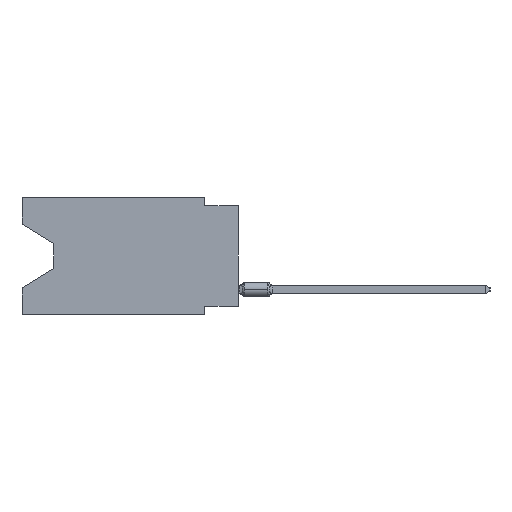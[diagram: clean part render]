
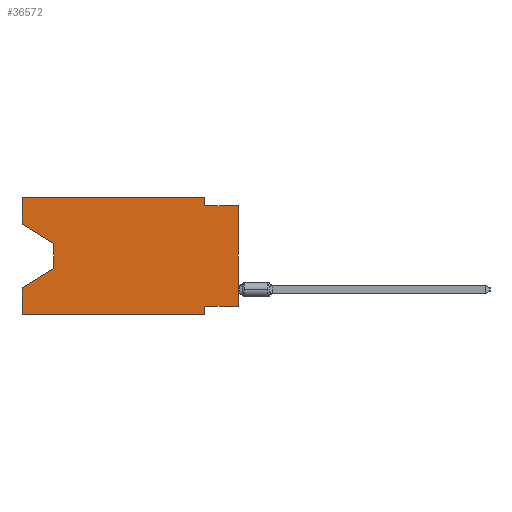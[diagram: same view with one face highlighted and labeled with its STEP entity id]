
A CAD part, left-side view. The second image highlights one B-rep face of the part: STEP entity #36572.
In plain terms, the highlighted planar face has unit normal (-1, 0, 0).
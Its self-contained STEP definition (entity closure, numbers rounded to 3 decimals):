
#488 = LINE ( 'NONE', #32282, #48132 ) ;
#2154 = LINE ( 'NONE', #9541, #48201 ) ;
#2436 = ORIENTED_EDGE ( 'NONE', *, *, #43017, .T. ) ;
#2719 = VECTOR ( 'NONE', #56922, 1000. ) ;
#3547 = CARTESIAN_POINT ( 'NONE',  ( 0., 0., -8.255 ) ) ;
#4063 = DIRECTION ( 'NONE',  ( 0., 0., -1. ) ) ;
#5570 = CARTESIAN_POINT ( 'NONE',  ( 0., 0., 0. ) ) ;
#5782 = CARTESIAN_POINT ( 'NONE',  ( 0., 13.97, -5.385 ) ) ;
#5794 = ORIENTED_EDGE ( 'NONE', *, *, #33889, .T. ) ;
#5879 = LINE ( 'NONE', #5570, #44792 ) ;
#5902 = VERTEX_POINT ( 'NONE', #37300 ) ;
#6176 = VERTEX_POINT ( 'NONE', #37143 ) ;
#6193 = VERTEX_POINT ( 'NONE', #56234 ) ;
#6718 = VECTOR ( 'NONE', #44140, 1000. ) ;
#6778 = VERTEX_POINT ( 'NONE', #57629 ) ;
#6966 = LINE ( 'NONE', #21487, #12558 ) ;
#7484 = CARTESIAN_POINT ( 'NONE',  ( 0., 2.54, -8.255 ) ) ;
#8605 = CARTESIAN_POINT ( 'NONE',  ( 0., 2.54, -8.89 ) ) ;
#9203 = LINE ( 'NONE', #8605, #39000 ) ;
#9541 = CARTESIAN_POINT ( 'NONE',  ( 0., 0., -0.635 ) ) ;
#11287 = VERTEX_POINT ( 'NONE', #26435 ) ;
#11572 = VECTOR ( 'NONE', #41340, 1000. ) ;
#11901 = VECTOR ( 'NONE', #38254, 1000. ) ;
#11938 = LINE ( 'NONE', #54308, #56886 ) ;
#12047 = DIRECTION ( 'NONE',  ( 0., -0.855, -0.519 ) ) ;
#12558 = VECTOR ( 'NONE', #39947, 1000. ) ;
#12720 = DIRECTION ( 'NONE',  ( 0., 0., -1. ) ) ;
#15863 = EDGE_CURVE ( 'NONE', #24066, #6193, #488, .T. ) ;
#17715 = VERTEX_POINT ( 'NONE', #45028 ) ;
#17745 = EDGE_CURVE ( 'NONE', #5902, #6778, #35042, .T. ) ;
#19246 = EDGE_CURVE ( 'NONE', #55940, #20017, #35339, .T. ) ;
#19556 = EDGE_CURVE ( 'NONE', #6193, #46070, #43899, .T. ) ;
#19627 = EDGE_CURVE ( 'NONE', #54800, #11287, #6966, .T. ) ;
#20017 = VERTEX_POINT ( 'NONE', #7484 ) ;
#21454 = AXIS2_PLACEMENT_3D ( 'NONE', #55140, #22735, #33334 ) ;
#21487 = CARTESIAN_POINT ( 'NONE',  ( 0., 16.383, 0. ) ) ;
#22234 = ORIENTED_EDGE ( 'NONE', *, *, #26419, .F. ) ;
#22735 = DIRECTION ( 'NONE',  ( 1., 0., 0. ) ) ;
#24066 = VERTEX_POINT ( 'NONE', #31237 ) ;
#24629 = DIRECTION ( 'NONE',  ( 0., 0., 1. ) ) ;
#26419 = EDGE_CURVE ( 'NONE', #5902, #24066, #47065, .T. ) ;
#26435 = CARTESIAN_POINT ( 'NONE',  ( 0., 16.383, -6.852 ) ) ;
#28792 = FACE_OUTER_BOUND ( 'NONE', #47687, .T. ) ;
#30637 = ORIENTED_EDGE ( 'NONE', *, *, #42861, .F. ) ;
#31160 = CARTESIAN_POINT ( 'NONE',  ( 0., 2.54, 0. ) ) ;
#31237 = CARTESIAN_POINT ( 'NONE',  ( 0., 16.383, 0. ) ) ;
#31656 = CARTESIAN_POINT ( 'NONE',  ( 0., 16.383, -8.89 ) ) ;
#32282 = CARTESIAN_POINT ( 'NONE',  ( 0., 16.383, 0. ) ) ;
#33334 = DIRECTION ( 'NONE',  ( 0., 0., -1. ) ) ;
#33889 = EDGE_CURVE ( 'NONE', #54800, #54374, #50740, .T. ) ;
#34258 = DIRECTION ( 'NONE',  ( 0., -1., 0. ) ) ;
#35042 = LINE ( 'NONE', #53526, #59930 ) ;
#35339 = LINE ( 'NONE', #3547, #6718 ) ;
#35821 = DIRECTION ( 'NONE',  ( 0., 0., -1. ) ) ;
#36210 = ORIENTED_EDGE ( 'NONE', *, *, #15863, .F. ) ;
#36572 = ADVANCED_FACE ( 'NONE', ( #28792 ), #36653, .F. ) ;
#36653 = PLANE ( 'NONE',  #21454 ) ;
#37143 = CARTESIAN_POINT ( 'NONE',  ( 0., 0., -0.635 ) ) ;
#37300 = CARTESIAN_POINT ( 'NONE',  ( 0., 16.383, -2.038 ) ) ;
#38254 = DIRECTION ( 'NONE',  ( 0., 0., 1. ) ) ;
#38451 = LINE ( 'NONE', #5782, #2719 ) ;
#39000 = VECTOR ( 'NONE', #4063, 1000. ) ;
#39947 = DIRECTION ( 'NONE',  ( 0., 0., 1. ) ) ;
#40046 = CARTESIAN_POINT ( 'NONE',  ( 0., 0., -8.255 ) ) ;
#41340 = DIRECTION ( 'NONE',  ( 0., -1., 0. ) ) ;
#41365 = DIRECTION ( 'NONE',  ( 0., -1., 0. ) ) ;
#42861 = EDGE_CURVE ( 'NONE', #20017, #54374, #9203, .T. ) ;
#43017 = EDGE_CURVE ( 'NONE', #55940, #6176, #5879, .T. ) ;
#43899 = LINE ( 'NONE', #31160, #45400 ) ;
#44140 = DIRECTION ( 'NONE',  ( 0., 1., 0. ) ) ;
#44792 = VECTOR ( 'NONE', #24629, 1000. ) ;
#45024 = CARTESIAN_POINT ( 'NONE',  ( 0., 2.54, -8.89 ) ) ;
#45028 = CARTESIAN_POINT ( 'NONE',  ( 0., 13.97, -5.385 ) ) ;
#45400 = VECTOR ( 'NONE', #12720, 1000. ) ;
#45781 = ORIENTED_EDGE ( 'NONE', *, *, #19246, .F. ) ;
#46070 = VERTEX_POINT ( 'NONE', #59064 ) ;
#46467 = CARTESIAN_POINT ( 'NONE',  ( 0., 16.383, 0. ) ) ;
#47065 = LINE ( 'NONE', #46467, #11901 ) ;
#47582 = ORIENTED_EDGE ( 'NONE', *, *, #19556, .F. ) ;
#47687 = EDGE_LOOP ( 'NONE', ( #55537, #50883, #51392, #55892, #5794, #30637, #45781, #2436, #52766, #47582, #36210, #22234 ) ) ;
#48132 = VECTOR ( 'NONE', #41365, 1000. ) ;
#48201 = VECTOR ( 'NONE', #34258, 1000. ) ;
#49802 = EDGE_CURVE ( 'NONE', #17715, #11287, #38451, .T. ) ;
#50362 = EDGE_CURVE ( 'NONE', #46070, #6176, #2154, .T. ) ;
#50648 = EDGE_CURVE ( 'NONE', #6778, #17715, #11938, .T. ) ;
#50740 = LINE ( 'NONE', #31656, #11572 ) ;
#50883 = ORIENTED_EDGE ( 'NONE', *, *, #50648, .T. ) ;
#51392 = ORIENTED_EDGE ( 'NONE', *, *, #49802, .T. ) ;
#52766 = ORIENTED_EDGE ( 'NONE', *, *, #50362, .F. ) ;
#53526 = CARTESIAN_POINT ( 'NONE',  ( 0., 16.383, -2.038 ) ) ;
#54308 = CARTESIAN_POINT ( 'NONE',  ( 0., 13.97, -3.505 ) ) ;
#54374 = VERTEX_POINT ( 'NONE', #45024 ) ;
#54800 = VERTEX_POINT ( 'NONE', #55765 ) ;
#55140 = CARTESIAN_POINT ( 'NONE',  ( 0., 16.383, 0. ) ) ;
#55537 = ORIENTED_EDGE ( 'NONE', *, *, #17745, .T. ) ;
#55765 = CARTESIAN_POINT ( 'NONE',  ( 0., 16.383, -8.89 ) ) ;
#55892 = ORIENTED_EDGE ( 'NONE', *, *, #19627, .F. ) ;
#55940 = VERTEX_POINT ( 'NONE', #40046 ) ;
#56234 = CARTESIAN_POINT ( 'NONE',  ( 0., 2.54, 0. ) ) ;
#56886 = VECTOR ( 'NONE', #35821, 1000. ) ;
#56922 = DIRECTION ( 'NONE',  ( 0., 0.855, -0.519 ) ) ;
#57629 = CARTESIAN_POINT ( 'NONE',  ( 0., 13.97, -3.505 ) ) ;
#59064 = CARTESIAN_POINT ( 'NONE',  ( 0., 2.54, -0.635 ) ) ;
#59930 = VECTOR ( 'NONE', #12047, 1000. ) ;
